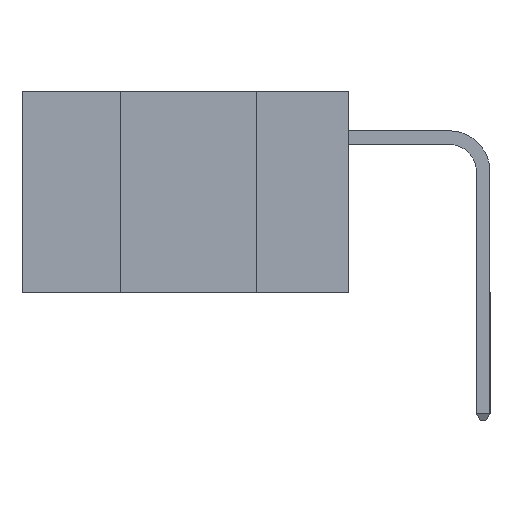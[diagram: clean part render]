
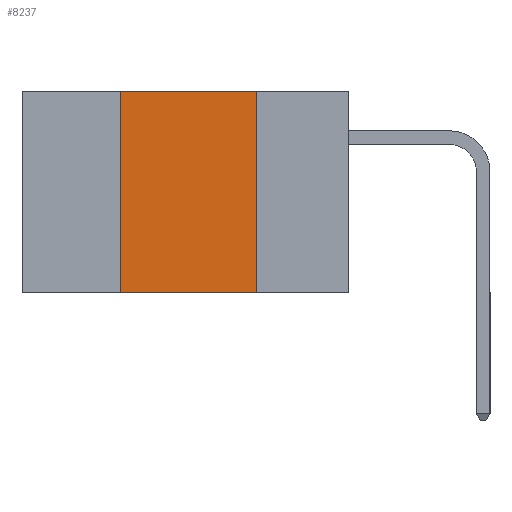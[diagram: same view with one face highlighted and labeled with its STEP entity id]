
A CAD part, left-side view. The second image highlights one B-rep face of the part: STEP entity #8237.
In plain terms, the highlighted planar face has unit normal (-1, 0, 0).
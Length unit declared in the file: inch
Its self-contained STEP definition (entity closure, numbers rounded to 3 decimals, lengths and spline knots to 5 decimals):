
#453 = VECTOR ( 'NONE', #3680, 39.37008 ) ;
#844 = EDGE_CURVE ( 'NONE', #4038, #889, #7744, .T. ) ;
#889 = VERTEX_POINT ( 'NONE', #3356 ) ;
#1260 = DIRECTION ( 'NONE',  ( 1., 0., 0. ) ) ;
#1509 = VECTOR ( 'NONE', #6839, 39.37008 ) ;
#1557 = VECTOR ( 'NONE', #5963, 39.37008 ) ;
#2266 = CARTESIAN_POINT ( 'NONE',  ( 0., 0.6, -0.37 ) ) ;
#2383 = CARTESIAN_POINT ( 'NONE',  ( 0., 0.42, 0. ) ) ;
#2574 = EDGE_LOOP ( 'NONE', ( #7106, #7117, #7157, #7208 ) ) ;
#2830 = DIRECTION ( 'NONE',  ( 0., -1., 0. ) ) ;
#2910 = VERTEX_POINT ( 'NONE', #2383 ) ;
#2954 = CARTESIAN_POINT ( 'NONE',  ( 0., 0.6, 0. ) ) ;
#3356 = CARTESIAN_POINT ( 'NONE',  ( 0., 0.17, -0.37 ) ) ;
#3443 = VERTEX_POINT ( 'NONE', #7766 ) ;
#3584 = LINE ( 'NONE', #5998, #1557 ) ;
#3680 = DIRECTION ( 'NONE',  ( 0., -1., 0. ) ) ;
#3761 = LINE ( 'NONE', #6575, #1509 ) ;
#4038 = VERTEX_POINT ( 'NONE', #5395 ) ;
#4203 = EDGE_CURVE ( 'NONE', #3443, #889, #3584, .T. ) ;
#4637 = AXIS2_PLACEMENT_3D ( 'NONE', #6808, #1260, #6193 ) ;
#5316 = FACE_OUTER_BOUND ( 'NONE', #2574, .T. ) ;
#5395 = CARTESIAN_POINT ( 'NONE',  ( 0., 0.42, -0.37 ) ) ;
#5963 = DIRECTION ( 'NONE',  ( 0., 0., -1. ) ) ;
#5998 = CARTESIAN_POINT ( 'NONE',  ( 0., 0.17, 0. ) ) ;
#6193 = DIRECTION ( 'NONE',  ( 0., 0., -1. ) ) ;
#6194 = LINE ( 'NONE', #2954, #453 ) ;
#6575 = CARTESIAN_POINT ( 'NONE',  ( 0., 0.42, 0. ) ) ;
#6808 = CARTESIAN_POINT ( 'NONE',  ( 0., 0.6, 0. ) ) ;
#6839 = DIRECTION ( 'NONE',  ( 0., 0., 1. ) ) ;
#6952 = EDGE_CURVE ( 'NONE', #4038, #2910, #3761, .T. ) ;
#7106 = ORIENTED_EDGE ( 'NONE', *, *, #4203, .F. ) ;
#7117 = ORIENTED_EDGE ( 'NONE', *, *, #8784, .F. ) ;
#7157 = ORIENTED_EDGE ( 'NONE', *, *, #6952, .F. ) ;
#7208 = ORIENTED_EDGE ( 'NONE', *, *, #844, .T. ) ;
#7744 = LINE ( 'NONE', #2266, #7951 ) ;
#7766 = CARTESIAN_POINT ( 'NONE',  ( 0., 0.17, 0. ) ) ;
#7951 = VECTOR ( 'NONE', #2830, 39.37008 ) ;
#8237 = ADVANCED_FACE ( 'NONE', ( #5316 ), #8656, .F. ) ;
#8656 = PLANE ( 'NONE',  #4637 ) ;
#8784 = EDGE_CURVE ( 'NONE', #2910, #3443, #6194, .T. ) ;
